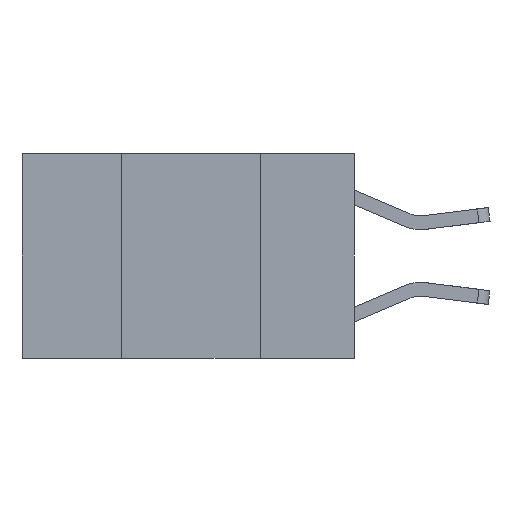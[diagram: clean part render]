
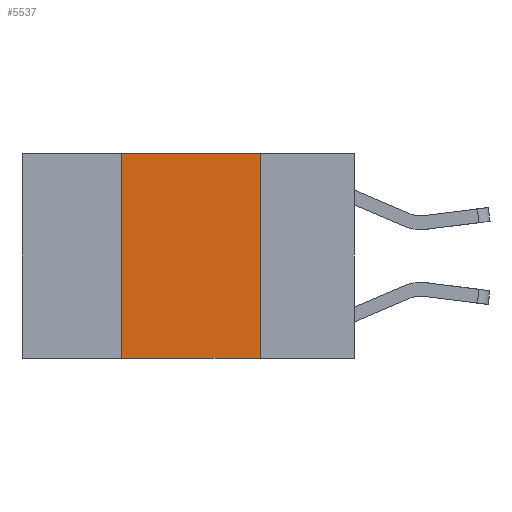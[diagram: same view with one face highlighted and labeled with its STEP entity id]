
A CAD part, left-side view. The second image highlights one B-rep face of the part: STEP entity #5537.
In plain terms, the highlighted planar face has unit normal (-1, 0, 0).
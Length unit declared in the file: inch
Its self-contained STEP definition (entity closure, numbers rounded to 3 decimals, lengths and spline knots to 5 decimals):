
#83 = ORIENTED_EDGE ( 'NONE', *, *, #6577, .T. ) ;
#99 = DIRECTION ( 'NONE',  ( 0., 0., 1. ) ) ;
#561 = ORIENTED_EDGE ( 'NONE', *, *, #890, .F. ) ;
#771 = LINE ( 'NONE', #8450, #10248 ) ;
#775 = CARTESIAN_POINT ( 'NONE',  ( 0., 0.42, -0.37 ) ) ;
#890 = EDGE_CURVE ( 'NONE', #3738, #5158, #1638, .T. ) ;
#1244 = DIRECTION ( 'NONE',  ( 1., 0., 0. ) ) ;
#1553 = AXIS2_PLACEMENT_3D ( 'NONE', #6774, #1244, #7709 ) ;
#1638 = LINE ( 'NONE', #6283, #8992 ) ;
#1754 = ORIENTED_EDGE ( 'NONE', *, *, #7196, .F. ) ;
#2047 = VECTOR ( 'NONE', #4979, 39.37008 ) ;
#2435 = ORIENTED_EDGE ( 'NONE', *, *, #4727, .F. ) ;
#3048 = PLANE ( 'NONE',  #1553 ) ;
#3738 = VERTEX_POINT ( 'NONE', #5306 ) ;
#4533 = LINE ( 'NONE', #11062, #6373 ) ;
#4727 = EDGE_CURVE ( 'NONE', #5158, #11239, #771, .T. ) ;
#4979 = DIRECTION ( 'NONE',  ( 0., -1., 0. ) ) ;
#5158 = VERTEX_POINT ( 'NONE', #8086 ) ;
#5306 = CARTESIAN_POINT ( 'NONE',  ( 0., 0.42, 0. ) ) ;
#5537 = ADVANCED_FACE ( 'NONE', ( #6551 ), #3048, .F. ) ;
#6283 = CARTESIAN_POINT ( 'NONE',  ( 0., 0.6, 0. ) ) ;
#6373 = VECTOR ( 'NONE', #99, 39.37008 ) ;
#6551 = FACE_OUTER_BOUND ( 'NONE', #8441, .T. ) ;
#6577 = EDGE_CURVE ( 'NONE', #11591, #11239, #11663, .T. ) ;
#6774 = CARTESIAN_POINT ( 'NONE',  ( 0., 0.6, 0. ) ) ;
#7196 = EDGE_CURVE ( 'NONE', #11591, #3738, #4533, .T. ) ;
#7709 = DIRECTION ( 'NONE',  ( 0., 0., -1. ) ) ;
#7849 = CARTESIAN_POINT ( 'NONE',  ( 0., 0.17, -0.37 ) ) ;
#8086 = CARTESIAN_POINT ( 'NONE',  ( 0., 0.17, 0. ) ) ;
#8441 = EDGE_LOOP ( 'NONE', ( #2435, #561, #1754, #83 ) ) ;
#8450 = CARTESIAN_POINT ( 'NONE',  ( 0., 0.17, 0. ) ) ;
#8699 = DIRECTION ( 'NONE',  ( 0., -1., 0. ) ) ;
#8992 = VECTOR ( 'NONE', #8699, 39.37008 ) ;
#9346 = DIRECTION ( 'NONE',  ( 0., 0., -1. ) ) ;
#10248 = VECTOR ( 'NONE', #9346, 39.37008 ) ;
#11062 = CARTESIAN_POINT ( 'NONE',  ( 0., 0.42, 0. ) ) ;
#11220 = CARTESIAN_POINT ( 'NONE',  ( 0., 0.6, -0.37 ) ) ;
#11239 = VERTEX_POINT ( 'NONE', #7849 ) ;
#11591 = VERTEX_POINT ( 'NONE', #775 ) ;
#11663 = LINE ( 'NONE', #11220, #2047 ) ;
